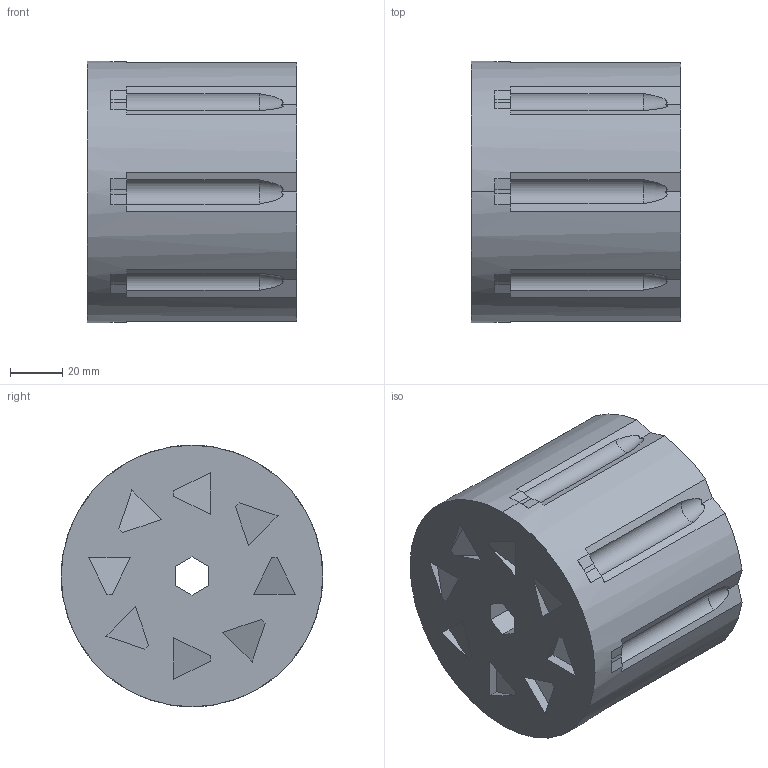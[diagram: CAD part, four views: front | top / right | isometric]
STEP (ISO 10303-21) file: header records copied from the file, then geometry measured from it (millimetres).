
FILE_DESCRIPTION (( 'STEP AP214' ), '1' );
FILE_NAME ('rotating cyilnder 5.56.STEP', '2025-05-18T10:58:25', ( '' ), ( '' ), 'SwSTEP 2.0', 'SolidWorks 2024', '' );
FILE_SCHEMA (( 'AUTOMOTIVE_DESIGN' ));
Length unit declared in the file: millimetre
Products named in the file (1): rotating cyilnder 5.56
Bounding box: 80 x 100 x 100 mm (x, y, z)
Volume: 593503.6 mm3; surface area: 49832.8 mm2
Topology: 1 solids, 1 shells, 138 faces, 360 edges, 240 vertices
Faces by surface type: plane 104, cylinder 26, torus 8
Entity records: 4591 total; most frequent: CARTESIAN_POINT 1107, ORIENTED_EDGE 720, DIRECTION 706, EDGE_CURVE 360, LINE 260, VECTOR 260, VERTEX_POINT 240, AXIS2_PLACEMENT_3D 223
